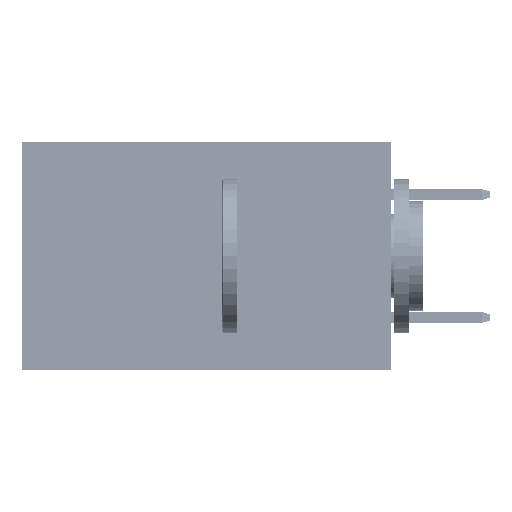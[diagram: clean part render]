
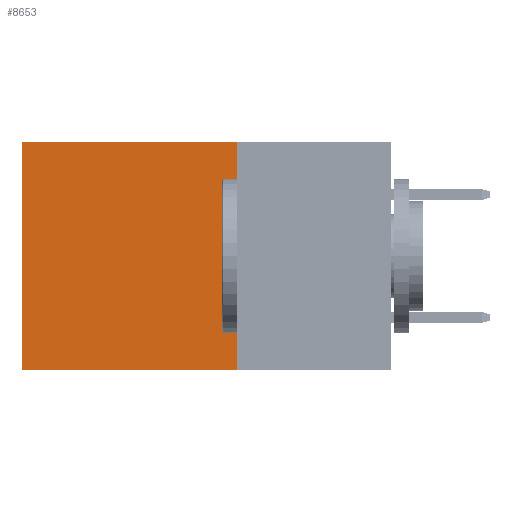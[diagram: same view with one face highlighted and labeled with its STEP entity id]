
A CAD part, left-side view. The second image highlights one B-rep face of the part: STEP entity #8653.
In plain terms, the highlighted planar face has unit normal (-1, 0, 0).
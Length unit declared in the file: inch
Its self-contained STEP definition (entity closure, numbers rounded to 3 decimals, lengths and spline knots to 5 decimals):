
#821 = EDGE_CURVE ( 'NONE', #11968, #30965, #20674, .T. ) ;
#1391 = LINE ( 'NONE', #10986, #28337 ) ;
#1566 = CARTESIAN_POINT ( 'NONE',  ( 0.2875, 0.6, 0. ) ) ;
#1626 = ORIENTED_EDGE ( 'NONE', *, *, #20165, .T. ) ;
#2036 = EDGE_CURVE ( 'NONE', #39932, #11968, #30220, .T. ) ;
#3358 = LINE ( 'NONE', #1566, #48023 ) ;
#4282 = DIRECTION ( 'NONE',  ( 0., 0., -1. ) ) ;
#6644 = CARTESIAN_POINT ( 'NONE',  ( 0.2875, 0.25, -0.37 ) ) ;
#8653 = ADVANCED_FACE ( 'NONE', ( #43135 ), #15897, .F. ) ;
#9064 = EDGE_LOOP ( 'NONE', ( #29730, #10605, #26320, #1626 ) ) ;
#10605 = ORIENTED_EDGE ( 'NONE', *, *, #821, .F. ) ;
#10654 = AXIS2_PLACEMENT_3D ( 'NONE', #33285, #25757, #4282 ) ;
#10986 = CARTESIAN_POINT ( 'NONE',  ( 0.2875, 0.25, 0. ) ) ;
#11968 = VERTEX_POINT ( 'NONE', #17310 ) ;
#14168 = VECTOR ( 'NONE', #36826, 39.37008 ) ;
#15315 = CARTESIAN_POINT ( 'NONE',  ( 0.2875, 0.25, 0. ) ) ;
#15897 = PLANE ( 'NONE',  #10654 ) ;
#17310 = CARTESIAN_POINT ( 'NONE',  ( 0.2875, 0.25, -0.37 ) ) ;
#18035 = DIRECTION ( 'NONE',  ( 0., 1., 0. ) ) ;
#19304 = VERTEX_POINT ( 'NONE', #28713 ) ;
#20165 = EDGE_CURVE ( 'NONE', #39932, #19304, #1391, .T. ) ;
#20258 = VECTOR ( 'NONE', #22156, 39.37008 ) ;
#20674 = LINE ( 'NONE', #6644, #14168 ) ;
#22156 = DIRECTION ( 'NONE',  ( 0., 0., -1. ) ) ;
#22532 = CARTESIAN_POINT ( 'NONE',  ( 0.2875, 0.25, 0. ) ) ;
#25757 = DIRECTION ( 'NONE',  ( 1., 0., 0. ) ) ;
#26320 = ORIENTED_EDGE ( 'NONE', *, *, #2036, .F. ) ;
#28337 = VECTOR ( 'NONE', #18035, 39.37008 ) ;
#28713 = CARTESIAN_POINT ( 'NONE',  ( 0.2875, 0.6, 0. ) ) ;
#29730 = ORIENTED_EDGE ( 'NONE', *, *, #40191, .T. ) ;
#30220 = LINE ( 'NONE', #22532, #20258 ) ;
#30965 = VERTEX_POINT ( 'NONE', #33992 ) ;
#33285 = CARTESIAN_POINT ( 'NONE',  ( 0.2875, 0.25, 0. ) ) ;
#33992 = CARTESIAN_POINT ( 'NONE',  ( 0.2875, 0.6, -0.37 ) ) ;
#35827 = DIRECTION ( 'NONE',  ( 0., 0., -1. ) ) ;
#36826 = DIRECTION ( 'NONE',  ( 0., 1., 0. ) ) ;
#39932 = VERTEX_POINT ( 'NONE', #15315 ) ;
#40191 = EDGE_CURVE ( 'NONE', #19304, #30965, #3358, .T. ) ;
#43135 = FACE_OUTER_BOUND ( 'NONE', #9064, .T. ) ;
#48023 = VECTOR ( 'NONE', #35827, 39.37008 ) ;
